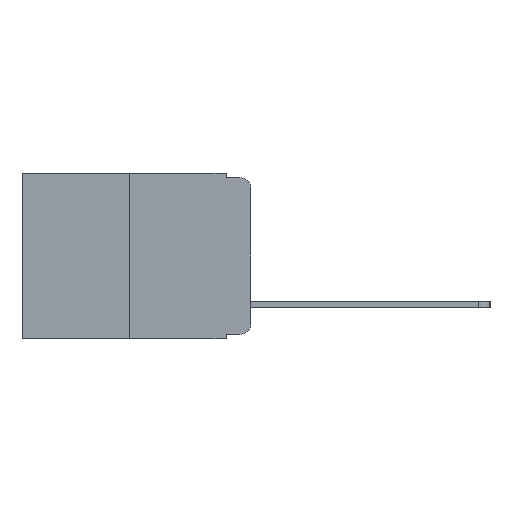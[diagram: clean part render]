
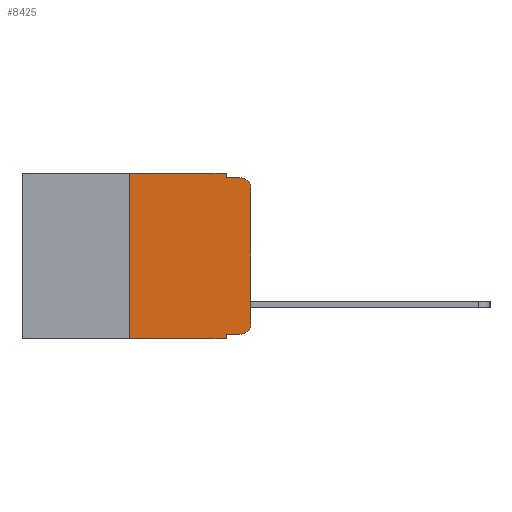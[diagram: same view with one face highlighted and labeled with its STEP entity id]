
A CAD part, left-side view. The second image highlights one B-rep face of the part: STEP entity #8425.
In plain terms, the highlighted planar face has unit normal (-1, 0, 0).
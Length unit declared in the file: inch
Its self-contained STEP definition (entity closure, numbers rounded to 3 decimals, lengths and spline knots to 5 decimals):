
#53 = CARTESIAN_POINT ( 'NONE',  ( 0., 0.02, -0.01 ) ) ;
#374 = DIRECTION ( 'NONE',  ( -1., 0., 0. ) ) ;
#391 = DIRECTION ( 'NONE',  ( 0., 0., -1. ) ) ;
#436 = CARTESIAN_POINT ( 'NONE',  ( 0., 0.02, -0.313 ) ) ;
#441 = VERTEX_POINT ( 'NONE', #6591 ) ;
#465 = VECTOR ( 'NONE', #9815, 39.37008 ) ;
#588 = VERTEX_POINT ( 'NONE', #7761 ) ;
#619 = VECTOR ( 'NONE', #6111, 39.37008 ) ;
#798 = VECTOR ( 'NONE', #6992, 39.37008 ) ;
#1059 = VERTEX_POINT ( 'NONE', #8229 ) ;
#1444 = DIRECTION ( 'NONE',  ( 0., -1., 0. ) ) ;
#1706 = EDGE_CURVE ( 'NONE', #5093, #1059, #3759, .T. ) ;
#2129 = VERTEX_POINT ( 'NONE', #6958 ) ;
#2778 = EDGE_CURVE ( 'NONE', #10564, #5615, #10850, .T. ) ;
#3125 = AXIS2_PLACEMENT_3D ( 'NONE', #7437, #7395, #7355 ) ;
#3198 = CARTESIAN_POINT ( 'NONE',  ( 0., 0.051, 0. ) ) ;
#3276 = DIRECTION ( 'NONE',  ( 0., 0., -1. ) ) ;
#3369 = EDGE_CURVE ( 'NONE', #588, #441, #9346, .T. ) ;
#3483 = EDGE_LOOP ( 'NONE', ( #5776, #5810, #5866, #6000, #6123, #6150, #6220, #6242, #6289, #6365 ) ) ;
#3759 = LINE ( 'NONE', #6960, #798 ) ;
#3802 = LINE ( 'NONE', #9952, #465 ) ;
#3976 = CARTESIAN_POINT ( 'NONE',  ( 0., 0.051, 0. ) ) ;
#4062 = VERTEX_POINT ( 'NONE', #7161 ) ;
#4306 = CARTESIAN_POINT ( 'NONE',  ( 0., 0., 0. ) ) ;
#4375 = PLANE ( 'NONE',  #6647 ) ;
#4839 = DIRECTION ( 'NONE',  ( 0., -1., 0. ) ) ;
#4878 = CARTESIAN_POINT ( 'NONE',  ( 0., 0.473, 0. ) ) ;
#5093 = VERTEX_POINT ( 'NONE', #10970 ) ;
#5184 = DIRECTION ( 'NONE',  ( 0., 0., 1. ) ) ;
#5203 = CARTESIAN_POINT ( 'NONE',  ( 0., 0.051, -0.01 ) ) ;
#5244 = DIRECTION ( 'NONE',  ( 1., 0., 0. ) ) ;
#5341 = EDGE_CURVE ( 'NONE', #5093, #10564, #3802, .T. ) ;
#5492 = EDGE_CURVE ( 'NONE', #5615, #5672, #9428, .T. ) ;
#5615 = VERTEX_POINT ( 'NONE', #3976 ) ;
#5672 = VERTEX_POINT ( 'NONE', #5203 ) ;
#5776 = ORIENTED_EDGE ( 'NONE', *, *, #6564, .T. ) ;
#5810 = ORIENTED_EDGE ( 'NONE', *, *, #7109, .T. ) ;
#5866 = ORIENTED_EDGE ( 'NONE', *, *, #7184, .F. ) ;
#5984 = LINE ( 'NONE', #11442, #619 ) ;
#6000 = ORIENTED_EDGE ( 'NONE', *, *, #5492, .F. ) ;
#6111 = DIRECTION ( 'NONE',  ( 0., -1., 0. ) ) ;
#6123 = ORIENTED_EDGE ( 'NONE', *, *, #2778, .F. ) ;
#6150 = ORIENTED_EDGE ( 'NONE', *, *, #5341, .F. ) ;
#6220 = ORIENTED_EDGE ( 'NONE', *, *, #1706, .T. ) ;
#6242 = ORIENTED_EDGE ( 'NONE', *, *, #10803, .F. ) ;
#6289 = ORIENTED_EDGE ( 'NONE', *, *, #7411, .T. ) ;
#6313 = VECTOR ( 'NONE', #11285, 39.37008 ) ;
#6344 = LINE ( 'NONE', #7015, #10395 ) ;
#6354 = AXIS2_PLACEMENT_3D ( 'NONE', #436, #374, #391 ) ;
#6365 = ORIENTED_EDGE ( 'NONE', *, *, #3369, .T. ) ;
#6564 = EDGE_CURVE ( 'NONE', #441, #4062, #10642, .T. ) ;
#6591 = CARTESIAN_POINT ( 'NONE',  ( 0., 0., -0.313 ) ) ;
#6647 = AXIS2_PLACEMENT_3D ( 'NONE', #7525, #5244, #10660 ) ;
#6725 = CARTESIAN_POINT ( 'NONE',  ( 0., 0.051, 0. ) ) ;
#6751 = VECTOR ( 'NONE', #4839, 39.37008 ) ;
#6958 = CARTESIAN_POINT ( 'NONE',  ( 0., 0.051, -0.333 ) ) ;
#6960 = CARTESIAN_POINT ( 'NONE',  ( 0., 0.473, -0.343 ) ) ;
#6992 = DIRECTION ( 'NONE',  ( 0., -1., 0. ) ) ;
#7015 = CARTESIAN_POINT ( 'NONE',  ( 0., 0.051, -0.333 ) ) ;
#7109 = EDGE_CURVE ( 'NONE', #4062, #7246, #10506, .T. ) ;
#7138 = VECTOR ( 'NONE', #3276, 39.37008 ) ;
#7161 = CARTESIAN_POINT ( 'NONE',  ( 0., 0., -0.03 ) ) ;
#7184 = EDGE_CURVE ( 'NONE', #5672, #7246, #5984, .T. ) ;
#7246 = VERTEX_POINT ( 'NONE', #53 ) ;
#7355 = DIRECTION ( 'NONE',  ( 0., 0., -1. ) ) ;
#7395 = DIRECTION ( 'NONE',  ( -1., 0., 0. ) ) ;
#7411 = EDGE_CURVE ( 'NONE', #2129, #588, #6344, .T. ) ;
#7437 = CARTESIAN_POINT ( 'NONE',  ( 0., 0.02, -0.03 ) ) ;
#7525 = CARTESIAN_POINT ( 'NONE',  ( 0., 0.473, 0. ) ) ;
#7761 = CARTESIAN_POINT ( 'NONE',  ( 0., 0.02, -0.333 ) ) ;
#8229 = CARTESIAN_POINT ( 'NONE',  ( 0., 0.051, -0.343 ) ) ;
#8425 = ADVANCED_FACE ( 'NONE', ( #10881 ), #4375, .F. ) ;
#9334 = CARTESIAN_POINT ( 'NONE',  ( 0., 0.25, 0. ) ) ;
#9346 = CIRCLE ( 'NONE', #6354, 0.02 ) ;
#9428 = LINE ( 'NONE', #6725, #7138 ) ;
#9815 = DIRECTION ( 'NONE',  ( 0., 0., 1. ) ) ;
#9952 = CARTESIAN_POINT ( 'NONE',  ( 0., 0.25, 0. ) ) ;
#10360 = LINE ( 'NONE', #3198, #6313 ) ;
#10395 = VECTOR ( 'NONE', #1444, 39.37008 ) ;
#10403 = VECTOR ( 'NONE', #5184, 39.37008 ) ;
#10506 = CIRCLE ( 'NONE', #3125, 0.02 ) ;
#10564 = VERTEX_POINT ( 'NONE', #9334 ) ;
#10642 = LINE ( 'NONE', #4306, #10403 ) ;
#10660 = DIRECTION ( 'NONE',  ( 0., 0., -1. ) ) ;
#10803 = EDGE_CURVE ( 'NONE', #2129, #1059, #10360, .T. ) ;
#10850 = LINE ( 'NONE', #4878, #6751 ) ;
#10881 = FACE_OUTER_BOUND ( 'NONE', #3483, .T. ) ;
#10970 = CARTESIAN_POINT ( 'NONE',  ( 0., 0.25, -0.343 ) ) ;
#11285 = DIRECTION ( 'NONE',  ( 0., 0., -1. ) ) ;
#11442 = CARTESIAN_POINT ( 'NONE',  ( 0., 0.051, -0.01 ) ) ;
